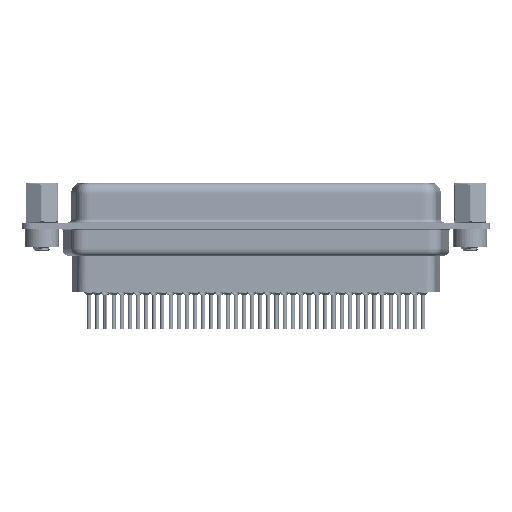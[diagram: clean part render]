
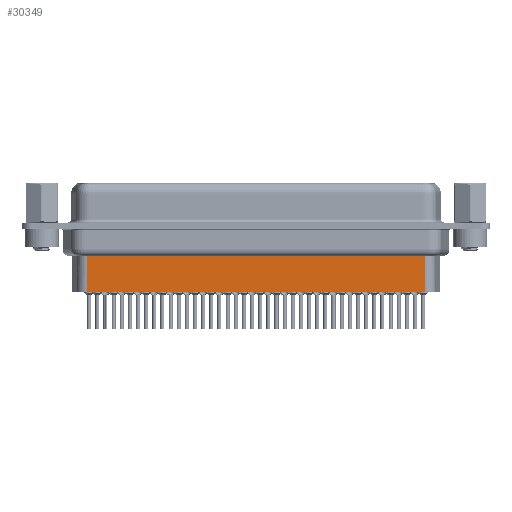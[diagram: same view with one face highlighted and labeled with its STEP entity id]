
A CAD part, front view. The second image highlights one B-rep face of the part: STEP entity #30349.
In plain terms, the highlighted planar face has unit normal (0, -1, 0).
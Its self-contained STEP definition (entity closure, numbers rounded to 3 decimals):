
#631 = DIRECTION ( 'NONE',  ( 0., 0., -1. ) ) ;
#1754 = VERTEX_POINT ( 'NONE', #8123 ) ;
#1919 = CARTESIAN_POINT ( 'NONE',  ( 56.794, -3.5, -9.85 ) ) ;
#2100 = CARTESIAN_POINT ( 'NONE',  ( 56.794, -3.5, -3.1 ) ) ;
#2485 = CARTESIAN_POINT ( 'NONE',  ( 6.459, -3.5, -4.097 ) ) ;
#3507 = VECTOR ( 'NONE', #39386, 1000. ) ;
#5988 = VECTOR ( 'NONE', #631, 1000. ) ;
#8123 = CARTESIAN_POINT ( 'NONE',  ( 6.706, -3.5, -9.85 ) ) ;
#8768 = VERTEX_POINT ( 'NONE', #1919 ) ;
#10086 = ORIENTED_EDGE ( 'NONE', *, *, #44514, .T. ) ;
#11871 = CARTESIAN_POINT ( 'NONE',  ( 6.706, -3.5, -9.85 ) ) ;
#12344 = AXIS2_PLACEMENT_3D ( 'NONE', #17407, #37356, #14011 ) ;
#13087 = VECTOR ( 'NONE', #43111, 1000. ) ;
#14011 = DIRECTION ( 'NONE',  ( 1., 0., 0. ) ) ;
#15762 = ORIENTED_EDGE ( 'NONE', *, *, #18702, .F. ) ;
#17298 = EDGE_CURVE ( 'NONE', #8768, #1754, #31535, .T. ) ;
#17407 = CARTESIAN_POINT ( 'NONE',  ( 6.706, -3.5, -3.1 ) ) ;
#18702 = EDGE_CURVE ( 'NONE', #33565, #8768, #38533, .T. ) ;
#21348 = PLANE ( 'NONE',  #12344 ) ;
#22494 = EDGE_CURVE ( 'NONE', #34440, #1754, #41010, .T. ) ;
#22656 = LINE ( 'NONE', #2485, #13087 ) ;
#30349 = ADVANCED_FACE ( 'NONE', ( #41810 ), #21348, .T. ) ;
#31268 = EDGE_LOOP ( 'NONE', ( #15762, #10086, #35648, #35284 ) ) ;
#31535 = LINE ( 'NONE', #11871, #3507 ) ;
#33565 = VERTEX_POINT ( 'NONE', #49559 ) ;
#34440 = VERTEX_POINT ( 'NONE', #34641 ) ;
#34641 = CARTESIAN_POINT ( 'NONE',  ( 6.706, -3.5, -4.097 ) ) ;
#35284 = ORIENTED_EDGE ( 'NONE', *, *, #17298, .F. ) ;
#35648 = ORIENTED_EDGE ( 'NONE', *, *, #22494, .T. ) ;
#36560 = CARTESIAN_POINT ( 'NONE',  ( 6.706, -3.5, -3.1 ) ) ;
#37356 = DIRECTION ( 'NONE',  ( 0., -1., 0. ) ) ;
#38533 = LINE ( 'NONE', #2100, #39625 ) ;
#39386 = DIRECTION ( 'NONE',  ( -1., 0., 0. ) ) ;
#39625 = VECTOR ( 'NONE', #46368, 1000. ) ;
#41010 = LINE ( 'NONE', #36560, #5988 ) ;
#41810 = FACE_OUTER_BOUND ( 'NONE', #31268, .T. ) ;
#43111 = DIRECTION ( 'NONE',  ( -1., 0., 0. ) ) ;
#44514 = EDGE_CURVE ( 'NONE', #33565, #34440, #22656, .T. ) ;
#46368 = DIRECTION ( 'NONE',  ( 0., 0., -1. ) ) ;
#49559 = CARTESIAN_POINT ( 'NONE',  ( 56.794, -3.5, -4.097 ) ) ;
